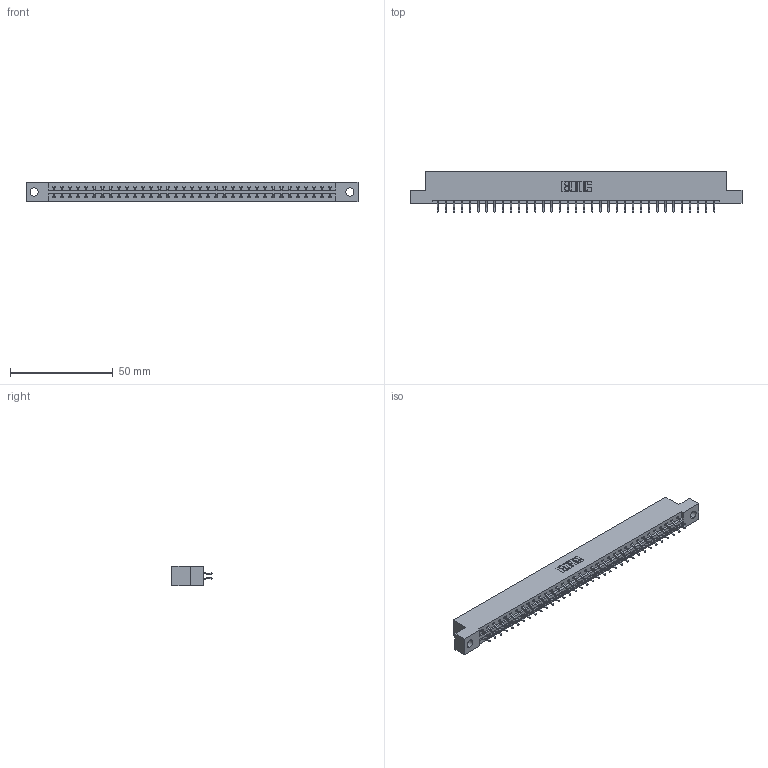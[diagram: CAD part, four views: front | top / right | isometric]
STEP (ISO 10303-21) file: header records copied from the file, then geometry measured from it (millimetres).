
FILE_DESCRIPTION (( 'STEP AP203' ), '1' );
FILE_NAME ('337-070-556-204.STEP', '2018-08-11T12:59:32', ( '' ), ( '' ), 'SwSTEP 2.0', 'SolidWorks 2016', '' );
FILE_SCHEMA (( 'CONFIG_CONTROL_DESIGN' ));
Length unit declared in the file: inch
Products named in the file (3): 337 Part_Flush Mounting Lugs - 0.156 Dia-TH; 345-292-001_556 Tail; 337-070-556-204
Assembly tree (71 placements, depth 2):
  337-070-556-204
    337 Part_Flush Mounting Lugs - 0.156 Dia-TH
    345-292-001_556 Tail  x70
Bounding box: 161.7 x 19.57 x 9.4 mm (x, y, z)
Volume: 16857 mm3; surface area: 18712.5 mm2
Topology: 71 solids, 71 shells, 4314 faces, 12841 edges, 8466 vertices
Faces by surface type: plane 3010, cylinder 1304
Entity records: 28265 total; most frequent: CARTESIAN_POINT 4782, ORIENTED_EDGE 4706, DIRECTION 4069, EDGE_CURVE 2353, LINE 2217, VECTOR 2217, VERTEX_POINT 1566, AXIS2_PLACEMENT_3D 926
